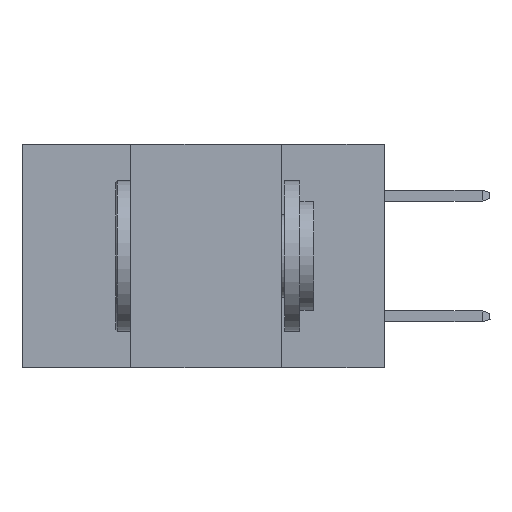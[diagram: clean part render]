
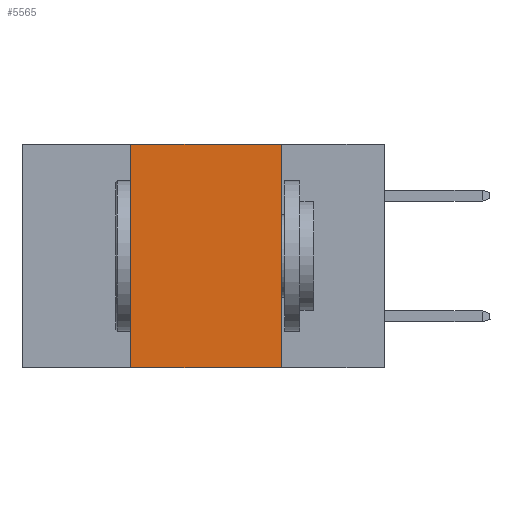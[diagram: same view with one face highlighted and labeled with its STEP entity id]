
A CAD part, left-side view. The second image highlights one B-rep face of the part: STEP entity #5565.
In plain terms, the highlighted planar face has unit normal (-1, 0, 0).
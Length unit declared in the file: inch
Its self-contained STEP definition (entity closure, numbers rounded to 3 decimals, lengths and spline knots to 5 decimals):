
#356 = VERTEX_POINT ( 'NONE', #13954 ) ;
#394 = LINE ( 'NONE', #6356, #13892 ) ;
#567 = ORIENTED_EDGE ( 'NONE', *, *, #16583, .F. ) ;
#772 = CARTESIAN_POINT ( 'NONE',  ( 0., 0.42, 0. ) ) ;
#936 = VECTOR ( 'NONE', #15153, 39.37008 ) ;
#1275 = LINE ( 'NONE', #3025, #14738 ) ;
#1511 = LINE ( 'NONE', #9973, #936 ) ;
#2065 = AXIS2_PLACEMENT_3D ( 'NONE', #5727, #7543, #19724 ) ;
#3025 = CARTESIAN_POINT ( 'NONE',  ( 0., 0.6, -0.37 ) ) ;
#3114 = EDGE_LOOP ( 'NONE', ( #8405, #13532, #567, #6445 ) ) ;
#4171 = CARTESIAN_POINT ( 'NONE',  ( 0., 0.6, 0. ) ) ;
#4440 = EDGE_CURVE ( 'NONE', #12540, #16858, #10379, .T. ) ;
#5565 = ADVANCED_FACE ( 'NONE', ( #14935 ), #17936, .F. ) ;
#5727 = CARTESIAN_POINT ( 'NONE',  ( 0., 0.6, 0. ) ) ;
#5929 = DIRECTION ( 'NONE',  ( 0., -1., 0. ) ) ;
#6356 = CARTESIAN_POINT ( 'NONE',  ( 0., 0.17, -0.37 ) ) ;
#6445 = ORIENTED_EDGE ( 'NONE', *, *, #15403, .T. ) ;
#7543 = DIRECTION ( 'NONE',  ( 1., 0., 0. ) ) ;
#8405 = ORIENTED_EDGE ( 'NONE', *, *, #9197, .F. ) ;
#8796 = VERTEX_POINT ( 'NONE', #10626 ) ;
#9197 = EDGE_CURVE ( 'NONE', #16858, #8796, #394, .T. ) ;
#9840 = VECTOR ( 'NONE', #5929, 39.37008 ) ;
#9973 = CARTESIAN_POINT ( 'NONE',  ( 0., 0.42, -0.37 ) ) ;
#10379 = LINE ( 'NONE', #4171, #9840 ) ;
#10626 = CARTESIAN_POINT ( 'NONE',  ( 0., 0.17, -0.37 ) ) ;
#10637 = CARTESIAN_POINT ( 'NONE',  ( 0., 0.17, 0. ) ) ;
#12540 = VERTEX_POINT ( 'NONE', #772 ) ;
#13367 = DIRECTION ( 'NONE',  ( 0., 0., -1. ) ) ;
#13532 = ORIENTED_EDGE ( 'NONE', *, *, #4440, .F. ) ;
#13892 = VECTOR ( 'NONE', #13367, 39.37008 ) ;
#13954 = CARTESIAN_POINT ( 'NONE',  ( 0., 0.42, -0.37 ) ) ;
#14738 = VECTOR ( 'NONE', #15281, 39.37008 ) ;
#14935 = FACE_OUTER_BOUND ( 'NONE', #3114, .T. ) ;
#15153 = DIRECTION ( 'NONE',  ( 0., 0., 1. ) ) ;
#15281 = DIRECTION ( 'NONE',  ( 0., -1., 0. ) ) ;
#15403 = EDGE_CURVE ( 'NONE', #356, #8796, #1275, .T. ) ;
#16583 = EDGE_CURVE ( 'NONE', #356, #12540, #1511, .T. ) ;
#16858 = VERTEX_POINT ( 'NONE', #10637 ) ;
#17936 = PLANE ( 'NONE',  #2065 ) ;
#19724 = DIRECTION ( 'NONE',  ( 0., 0., -1. ) ) ;
